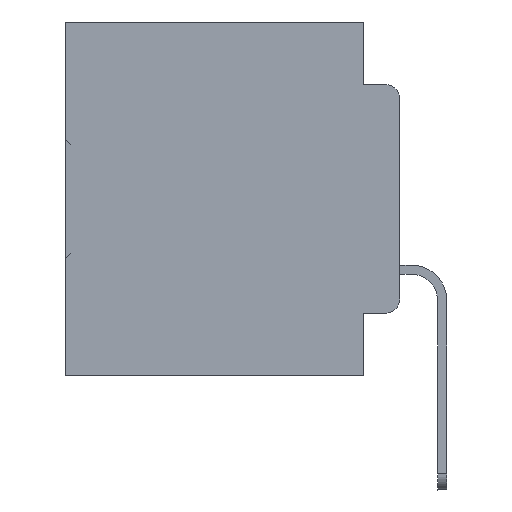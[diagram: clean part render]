
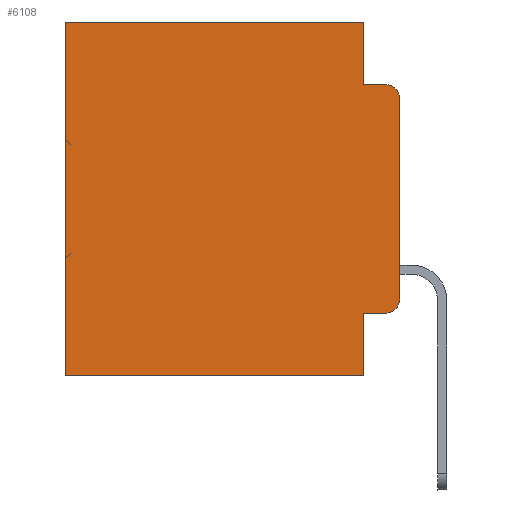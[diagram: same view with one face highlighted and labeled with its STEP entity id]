
A CAD part, left-side view. The second image highlights one B-rep face of the part: STEP entity #6108.
In plain terms, the highlighted planar face has unit normal (-1, 0, 0).
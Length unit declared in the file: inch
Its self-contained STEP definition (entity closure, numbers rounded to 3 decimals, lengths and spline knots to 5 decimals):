
#143 = DIRECTION ( 'NONE',  ( 0., -1., 0. ) ) ;
#529 = DIRECTION ( 'NONE',  ( 0., -1., 0. ) ) ;
#2683 = LINE ( 'NONE', #20250, #10660 ) ;
#3231 = DIRECTION ( 'NONE',  ( 0., 0., -1. ) ) ;
#3255 = VERTEX_POINT ( 'NONE', #21775 ) ;
#3332 = DIRECTION ( 'NONE',  ( 0., 0., -1. ) ) ;
#3416 = AXIS2_PLACEMENT_3D ( 'NONE', #18421, #29527, #27114 ) ;
#4317 = EDGE_CURVE ( 'NONE', #12556, #30707, #31621, .T. ) ;
#4376 = CARTESIAN_POINT ( 'NONE',  ( 0.298, 0., 0. ) ) ;
#4817 = EDGE_CURVE ( 'NONE', #7398, #12029, #27058, .T. ) ;
#5462 = VERTEX_POINT ( 'NONE', #25031 ) ;
#5659 = CARTESIAN_POINT ( 'NONE',  ( 0.298, 0.02, -0.4115 ) ) ;
#6066 = CARTESIAN_POINT ( 'NONE',  ( 0.298, 0.051, -0.4115 ) ) ;
#6108 = ADVANCED_FACE ( 'NONE', ( #9909 ), #27298, .F. ) ;
#7330 = DIRECTION ( 'NONE',  ( 0., 0., -1. ) ) ;
#7398 = VERTEX_POINT ( 'NONE', #5659 ) ;
#7544 = CARTESIAN_POINT ( 'NONE',  ( 0.298, 0.051, -0.0885 ) ) ;
#7635 = VECTOR ( 'NONE', #143, 39.37008 ) ;
#7687 = DIRECTION ( 'NONE',  ( 1., 0., 0. ) ) ;
#8640 = ORIENTED_EDGE ( 'NONE', *, *, #19040, .F. ) ;
#8696 = AXIS2_PLACEMENT_3D ( 'NONE', #4376, #7687, #7330 ) ;
#9696 = EDGE_CURVE ( 'NONE', #22607, #3255, #14617, .T. ) ;
#9909 = FACE_OUTER_BOUND ( 'NONE', #30576, .T. ) ;
#10176 = EDGE_CURVE ( 'NONE', #12485, #5462, #14572, .T. ) ;
#10441 = ORIENTED_EDGE ( 'NONE', *, *, #27181, .T. ) ;
#10660 = VECTOR ( 'NONE', #3231, 39.37008 ) ;
#11010 = DIRECTION ( 'NONE',  ( 0., 0., -1. ) ) ;
#11811 = CARTESIAN_POINT ( 'NONE',  ( 0.298, 0., -0.5 ) ) ;
#12029 = VERTEX_POINT ( 'NONE', #18690 ) ;
#12271 = ORIENTED_EDGE ( 'NONE', *, *, #4317, .F. ) ;
#12378 = DIRECTION ( 'NONE',  ( 0., 1., 0. ) ) ;
#12485 = VERTEX_POINT ( 'NONE', #7544 ) ;
#12556 = VERTEX_POINT ( 'NONE', #14360 ) ;
#12940 = ORIENTED_EDGE ( 'NONE', *, *, #28466, .F. ) ;
#13081 = CIRCLE ( 'NONE', #26679, 0.02 ) ;
#14028 = ORIENTED_EDGE ( 'NONE', *, *, #28942, .F. ) ;
#14187 = ORIENTED_EDGE ( 'NONE', *, *, #23606, .T. ) ;
#14360 = CARTESIAN_POINT ( 'NONE',  ( 0.298, 0.051, -0.5 ) ) ;
#14572 = LINE ( 'NONE', #34375, #23650 ) ;
#14617 = LINE ( 'NONE', #34790, #27268 ) ;
#15014 = VECTOR ( 'NONE', #23840, 39.37008 ) ;
#15850 = VERTEX_POINT ( 'NONE', #26755 ) ;
#16378 = LINE ( 'NONE', #28202, #16868 ) ;
#16746 = CARTESIAN_POINT ( 'NONE',  ( 0.298, 0.02, -0.1085 ) ) ;
#16868 = VECTOR ( 'NONE', #11010, 39.37008 ) ;
#17262 = VERTEX_POINT ( 'NONE', #33402 ) ;
#18421 = CARTESIAN_POINT ( 'NONE',  ( 0.298, 0.02, -0.3915 ) ) ;
#18690 = CARTESIAN_POINT ( 'NONE',  ( 0.298, 0., -0.3915 ) ) ;
#19040 = EDGE_CURVE ( 'NONE', #15850, #12029, #16378, .T. ) ;
#19575 = ORIENTED_EDGE ( 'NONE', *, *, #9696, .T. ) ;
#19616 = CARTESIAN_POINT ( 'NONE',  ( 0.298, 0.051, 0. ) ) ;
#19802 = VECTOR ( 'NONE', #3332, 39.37008 ) ;
#20250 = CARTESIAN_POINT ( 'NONE',  ( 0.298, 0.473, 0. ) ) ;
#20625 = DIRECTION ( 'NONE',  ( 0., 0., -1. ) ) ;
#21775 = CARTESIAN_POINT ( 'NONE',  ( 0.298, 0.473, 0. ) ) ;
#22566 = EDGE_CURVE ( 'NONE', #3255, #30707, #2683, .T. ) ;
#22607 = VERTEX_POINT ( 'NONE', #26676 ) ;
#22953 = LINE ( 'NONE', #19616, #19802 ) ;
#23606 = EDGE_CURVE ( 'NONE', #15850, #5462, #13081, .T. ) ;
#23650 = VECTOR ( 'NONE', #529, 39.37008 ) ;
#23840 = DIRECTION ( 'NONE',  ( 0., 1., 0. ) ) ;
#25031 = CARTESIAN_POINT ( 'NONE',  ( 0.298, 0.02, -0.0885 ) ) ;
#26352 = VECTOR ( 'NONE', #20625, 39.37008 ) ;
#26676 = CARTESIAN_POINT ( 'NONE',  ( 0.298, 0.051, 0. ) ) ;
#26679 = AXIS2_PLACEMENT_3D ( 'NONE', #16746, #27679, #36192 ) ;
#26755 = CARTESIAN_POINT ( 'NONE',  ( 0.298, 0., -0.1085 ) ) ;
#27058 = CIRCLE ( 'NONE', #3416, 0.02 ) ;
#27114 = DIRECTION ( 'NONE',  ( 0., 0., -1. ) ) ;
#27181 = EDGE_CURVE ( 'NONE', #17262, #7398, #31404, .T. ) ;
#27268 = VECTOR ( 'NONE', #12378, 39.37008 ) ;
#27298 = PLANE ( 'NONE',  #8696 ) ;
#27597 = ORIENTED_EDGE ( 'NONE', *, *, #22566, .T. ) ;
#27679 = DIRECTION ( 'NONE',  ( -1., 0., 0. ) ) ;
#28202 = CARTESIAN_POINT ( 'NONE',  ( 0.298, 0., 0. ) ) ;
#28466 = EDGE_CURVE ( 'NONE', #17262, #12556, #22953, .T. ) ;
#28758 = LINE ( 'NONE', #31739, #26352 ) ;
#28942 = EDGE_CURVE ( 'NONE', #22607, #12485, #28758, .T. ) ;
#29527 = DIRECTION ( 'NONE',  ( -1., 0., 0. ) ) ;
#30576 = EDGE_LOOP ( 'NONE', ( #8640, #14187, #32898, #14028, #19575, #27597, #12271, #12940, #10441, #36350 ) ) ;
#30707 = VERTEX_POINT ( 'NONE', #32600 ) ;
#31404 = LINE ( 'NONE', #6066, #7635 ) ;
#31621 = LINE ( 'NONE', #11811, #15014 ) ;
#31739 = CARTESIAN_POINT ( 'NONE',  ( 0.298, 0.051, 0. ) ) ;
#32600 = CARTESIAN_POINT ( 'NONE',  ( 0.298, 0.473, -0.5 ) ) ;
#32898 = ORIENTED_EDGE ( 'NONE', *, *, #10176, .F. ) ;
#33402 = CARTESIAN_POINT ( 'NONE',  ( 0.298, 0.051, -0.4115 ) ) ;
#34375 = CARTESIAN_POINT ( 'NONE',  ( 0.298, 0.051, -0.0885 ) ) ;
#34790 = CARTESIAN_POINT ( 'NONE',  ( 0.298, 0., 0. ) ) ;
#36192 = DIRECTION ( 'NONE',  ( 0., 0., -1. ) ) ;
#36350 = ORIENTED_EDGE ( 'NONE', *, *, #4817, .T. ) ;
